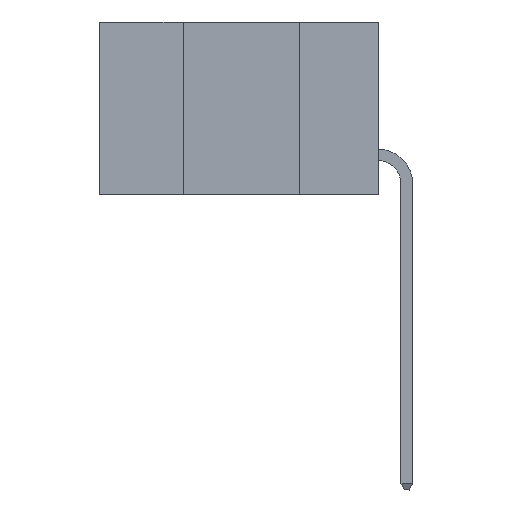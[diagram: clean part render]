
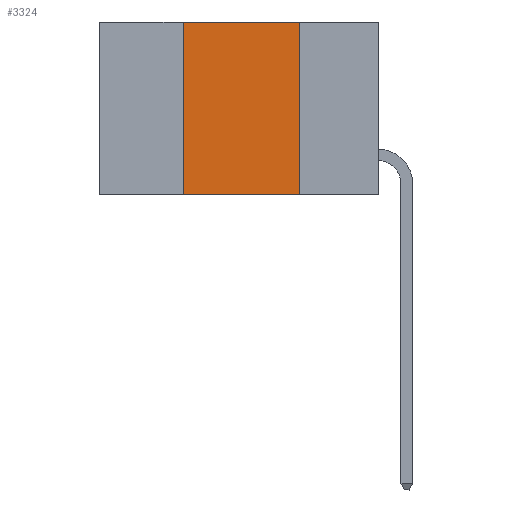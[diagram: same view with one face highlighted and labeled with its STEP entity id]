
A CAD part, left-side view. The second image highlights one B-rep face of the part: STEP entity #3324.
In plain terms, the highlighted planar face has unit normal (-1, 0, 0).
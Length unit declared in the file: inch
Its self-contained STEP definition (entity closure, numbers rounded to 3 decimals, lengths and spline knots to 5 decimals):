
#377 = VERTEX_POINT ( 'NONE', #2496 ) ;
#532 = EDGE_CURVE ( 'NONE', #1643, #12080, #9571, .T. ) ;
#684 = DIRECTION ( 'NONE',  ( 0., 0., 1. ) ) ;
#861 = CARTESIAN_POINT ( 'NONE',  ( 0., 0.17, 0. ) ) ;
#951 = VECTOR ( 'NONE', #6308, 39.37008 ) ;
#1418 = AXIS2_PLACEMENT_3D ( 'NONE', #4743, #1441, #3739 ) ;
#1441 = DIRECTION ( 'NONE',  ( 1., 0., 0. ) ) ;
#1643 = VERTEX_POINT ( 'NONE', #861 ) ;
#1871 = VECTOR ( 'NONE', #684, 39.37008 ) ;
#2274 = VERTEX_POINT ( 'NONE', #13951 ) ;
#2496 = CARTESIAN_POINT ( 'NONE',  ( 0., 0.42, 0. ) ) ;
#2526 = LINE ( 'NONE', #7357, #10934 ) ;
#2971 = FACE_OUTER_BOUND ( 'NONE', #11154, .T. ) ;
#3324 = ADVANCED_FACE ( 'NONE', ( #2971 ), #4791, .F. ) ;
#3508 = CARTESIAN_POINT ( 'NONE',  ( 0., 0.6, -0.37 ) ) ;
#3739 = DIRECTION ( 'NONE',  ( 0., 0., -1. ) ) ;
#4161 = ORIENTED_EDGE ( 'NONE', *, *, #9896, .F. ) ;
#4171 = ORIENTED_EDGE ( 'NONE', *, *, #12494, .F. ) ;
#4743 = CARTESIAN_POINT ( 'NONE',  ( 0., 0.6, 0. ) ) ;
#4791 = PLANE ( 'NONE',  #1418 ) ;
#6308 = DIRECTION ( 'NONE',  ( 0., 0., -1. ) ) ;
#6666 = DIRECTION ( 'NONE',  ( 0., -1., 0. ) ) ;
#7357 = CARTESIAN_POINT ( 'NONE',  ( 0., 0.6, 0. ) ) ;
#8463 = CARTESIAN_POINT ( 'NONE',  ( 0., 0.17, 0. ) ) ;
#8776 = LINE ( 'NONE', #12704, #1871 ) ;
#9571 = LINE ( 'NONE', #8463, #951 ) ;
#9896 = EDGE_CURVE ( 'NONE', #377, #1643, #2526, .T. ) ;
#10934 = VECTOR ( 'NONE', #6666, 39.37008 ) ;
#11012 = CARTESIAN_POINT ( 'NONE',  ( 0., 0.17, -0.37 ) ) ;
#11154 = EDGE_LOOP ( 'NONE', ( #13522, #4161, #4171, #11439 ) ) ;
#11439 = ORIENTED_EDGE ( 'NONE', *, *, #13396, .T. ) ;
#11651 = LINE ( 'NONE', #3508, #11988 ) ;
#11988 = VECTOR ( 'NONE', #13365, 39.37008 ) ;
#12080 = VERTEX_POINT ( 'NONE', #11012 ) ;
#12494 = EDGE_CURVE ( 'NONE', #2274, #377, #8776, .T. ) ;
#12704 = CARTESIAN_POINT ( 'NONE',  ( 0., 0.42, 0. ) ) ;
#13365 = DIRECTION ( 'NONE',  ( 0., -1., 0. ) ) ;
#13396 = EDGE_CURVE ( 'NONE', #2274, #12080, #11651, .T. ) ;
#13522 = ORIENTED_EDGE ( 'NONE', *, *, #532, .F. ) ;
#13951 = CARTESIAN_POINT ( 'NONE',  ( 0., 0.42, -0.37 ) ) ;
